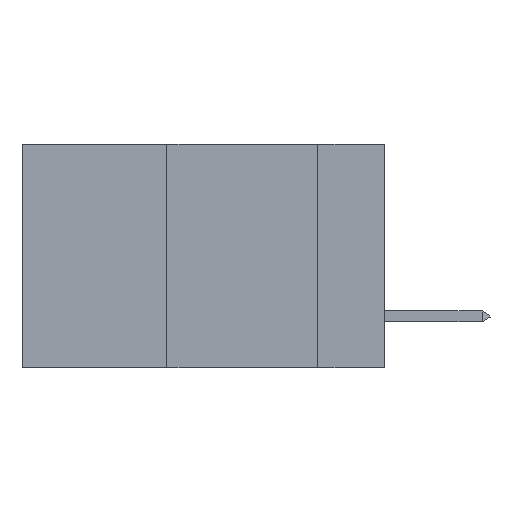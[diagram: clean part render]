
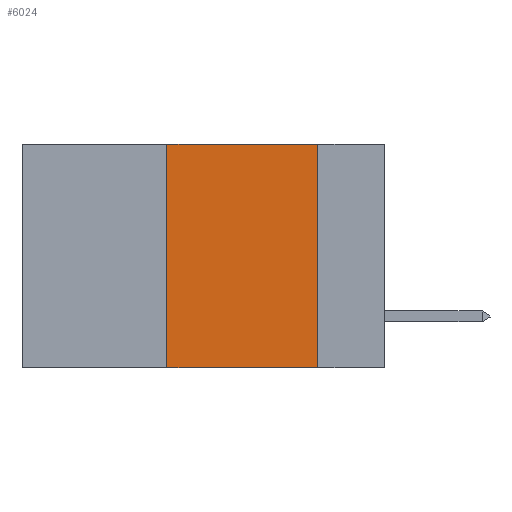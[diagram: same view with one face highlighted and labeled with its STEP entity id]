
A CAD part, left-side view. The second image highlights one B-rep face of the part: STEP entity #6024.
In plain terms, the highlighted planar face has unit normal (-1, 0, 0).
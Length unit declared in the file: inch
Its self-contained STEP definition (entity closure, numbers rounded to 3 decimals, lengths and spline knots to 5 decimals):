
#718 = EDGE_CURVE ( 'NONE', #12548, #14571, #7929, .T. ) ;
#887 = VERTEX_POINT ( 'NONE', #4921 ) ;
#965 = ORIENTED_EDGE ( 'NONE', *, *, #1623, .F. ) ;
#1623 = EDGE_CURVE ( 'NONE', #887, #9694, #6514, .T. ) ;
#1739 = VECTOR ( 'NONE', #5223, 39.37008 ) ;
#3058 = CARTESIAN_POINT ( 'NONE',  ( 0., 0.11, -0.37 ) ) ;
#3160 = EDGE_CURVE ( 'NONE', #9694, #12548, #7447, .T. ) ;
#3462 = VECTOR ( 'NONE', #12761, 39.37008 ) ;
#3764 = CARTESIAN_POINT ( 'NONE',  ( 0., 0.6, 0. ) ) ;
#4921 = CARTESIAN_POINT ( 'NONE',  ( 0., 0.36, -0.37 ) ) ;
#5163 = DIRECTION ( 'NONE',  ( 0., -1., 0. ) ) ;
#5223 = DIRECTION ( 'NONE',  ( 0., 0., 1. ) ) ;
#5944 = EDGE_CURVE ( 'NONE', #887, #14571, #15594, .T. ) ;
#6024 = ADVANCED_FACE ( 'NONE', ( #13199 ), #14215, .F. ) ;
#6514 = LINE ( 'NONE', #7868, #1739 ) ;
#6665 = DIRECTION ( 'NONE',  ( 0., 0., -1. ) ) ;
#7044 = VECTOR ( 'NONE', #5163, 39.37008 ) ;
#7447 = LINE ( 'NONE', #3764, #7044 ) ;
#7868 = CARTESIAN_POINT ( 'NONE',  ( 0., 0.36, 0. ) ) ;
#7929 = LINE ( 'NONE', #9772, #8321 ) ;
#8134 = CARTESIAN_POINT ( 'NONE',  ( 0., 0.6, 0. ) ) ;
#8321 = VECTOR ( 'NONE', #13450, 39.37008 ) ;
#9133 = ORIENTED_EDGE ( 'NONE', *, *, #3160, .F. ) ;
#9198 = CARTESIAN_POINT ( 'NONE',  ( 0., 0.36, 0. ) ) ;
#9410 = DIRECTION ( 'NONE',  ( 1., 0., 0. ) ) ;
#9694 = VERTEX_POINT ( 'NONE', #9198 ) ;
#9772 = CARTESIAN_POINT ( 'NONE',  ( 0., 0.11, 0. ) ) ;
#10612 = AXIS2_PLACEMENT_3D ( 'NONE', #8134, #9410, #6665 ) ;
#12411 = EDGE_LOOP ( 'NONE', ( #13952, #9133, #965, #13823 ) ) ;
#12548 = VERTEX_POINT ( 'NONE', #13915 ) ;
#12761 = DIRECTION ( 'NONE',  ( 0., -1., 0. ) ) ;
#13199 = FACE_OUTER_BOUND ( 'NONE', #12411, .T. ) ;
#13450 = DIRECTION ( 'NONE',  ( 0., 0., -1. ) ) ;
#13823 = ORIENTED_EDGE ( 'NONE', *, *, #5944, .T. ) ;
#13915 = CARTESIAN_POINT ( 'NONE',  ( 0., 0.11, 0. ) ) ;
#13952 = ORIENTED_EDGE ( 'NONE', *, *, #718, .F. ) ;
#14048 = CARTESIAN_POINT ( 'NONE',  ( 0., 0.6, -0.37 ) ) ;
#14215 = PLANE ( 'NONE',  #10612 ) ;
#14571 = VERTEX_POINT ( 'NONE', #3058 ) ;
#15594 = LINE ( 'NONE', #14048, #3462 ) ;
